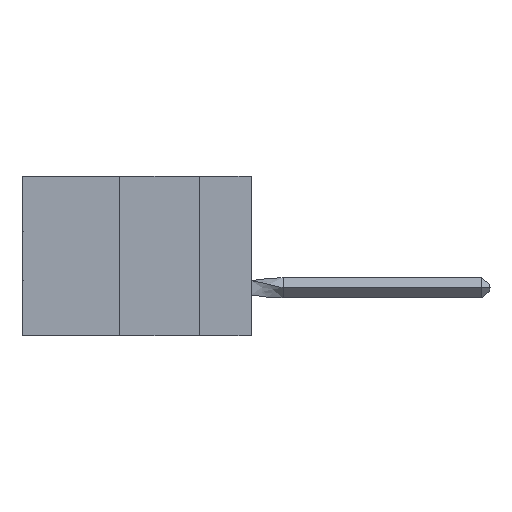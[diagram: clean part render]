
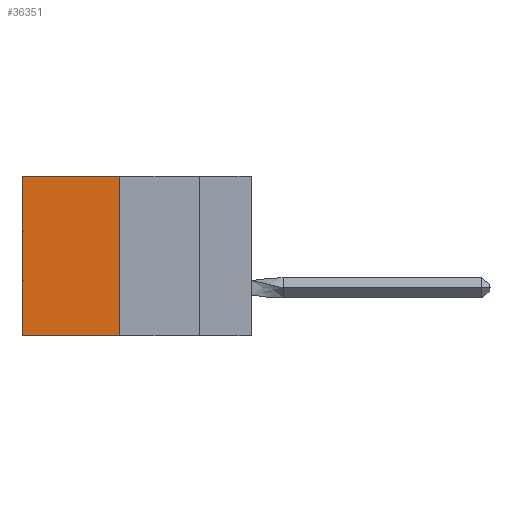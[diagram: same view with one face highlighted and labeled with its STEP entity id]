
A CAD part, left-side view. The second image highlights one B-rep face of the part: STEP entity #36351.
In plain terms, the highlighted planar face has unit normal (-1, 0, 0).
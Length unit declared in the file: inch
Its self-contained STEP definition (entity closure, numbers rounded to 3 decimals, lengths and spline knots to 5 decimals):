
#51 = CARTESIAN_POINT ( 'NONE',  ( 0.305, 0.72, -0.5 ) ) ;
#473 = EDGE_CURVE ( 'NONE', #9166, #6131, #24667, .T. ) ;
#812 = FACE_OUTER_BOUND ( 'NONE', #2274, .T. ) ;
#2274 = EDGE_LOOP ( 'NONE', ( #14143, #43478, #26600, #22146 ) ) ;
#3530 = CARTESIAN_POINT ( 'NONE',  ( 0.305, 0.413, 0. ) ) ;
#4498 = LINE ( 'NONE', #8764, #38368 ) ;
#6131 = VERTEX_POINT ( 'NONE', #32258 ) ;
#6392 = AXIS2_PLACEMENT_3D ( 'NONE', #42616, #46285, #28176 ) ;
#6401 = VERTEX_POINT ( 'NONE', #26428 ) ;
#6738 = DIRECTION ( 'NONE',  ( 0., 1., 0. ) ) ;
#6821 = LINE ( 'NONE', #3530, #35655 ) ;
#8726 = EDGE_CURVE ( 'NONE', #13160, #6131, #26101, .T. ) ;
#8764 = CARTESIAN_POINT ( 'NONE',  ( 0.305, 0.413, -0.5 ) ) ;
#9166 = VERTEX_POINT ( 'NONE', #20437 ) ;
#9474 = EDGE_CURVE ( 'NONE', #6401, #13160, #6821, .T. ) ;
#13160 = VERTEX_POINT ( 'NONE', #33735 ) ;
#13871 = VECTOR ( 'NONE', #6738, 39.37008 ) ;
#14143 = ORIENTED_EDGE ( 'NONE', *, *, #8726, .T. ) ;
#16470 = VECTOR ( 'NONE', #25133, 39.37008 ) ;
#17262 = CARTESIAN_POINT ( 'NONE',  ( 0.305, 0.413, -0.5 ) ) ;
#20437 = CARTESIAN_POINT ( 'NONE',  ( 0.305, 0.413, -0.5 ) ) ;
#22146 = ORIENTED_EDGE ( 'NONE', *, *, #9474, .T. ) ;
#24667 = LINE ( 'NONE', #17262, #13871 ) ;
#25133 = DIRECTION ( 'NONE',  ( 0., 0., -1. ) ) ;
#26101 = LINE ( 'NONE', #51, #16470 ) ;
#26428 = CARTESIAN_POINT ( 'NONE',  ( 0.305, 0.413, 0. ) ) ;
#26600 = ORIENTED_EDGE ( 'NONE', *, *, #39027, .F. ) ;
#28176 = DIRECTION ( 'NONE',  ( 0., 0., -1. ) ) ;
#32258 = CARTESIAN_POINT ( 'NONE',  ( 0.305, 0.72, -0.5 ) ) ;
#33735 = CARTESIAN_POINT ( 'NONE',  ( 0.305, 0.72, 0. ) ) ;
#35655 = VECTOR ( 'NONE', #43355, 39.37008 ) ;
#36351 = ADVANCED_FACE ( 'NONE', ( #812 ), #38954, .F. ) ;
#38368 = VECTOR ( 'NONE', #45007, 39.37008 ) ;
#38954 = PLANE ( 'NONE',  #6392 ) ;
#39027 = EDGE_CURVE ( 'NONE', #6401, #9166, #4498, .T. ) ;
#42616 = CARTESIAN_POINT ( 'NONE',  ( 0.305, 0.413, -0.5 ) ) ;
#43355 = DIRECTION ( 'NONE',  ( 0., 1., 0. ) ) ;
#43478 = ORIENTED_EDGE ( 'NONE', *, *, #473, .F. ) ;
#45007 = DIRECTION ( 'NONE',  ( 0., 0., -1. ) ) ;
#46285 = DIRECTION ( 'NONE',  ( 1., 0., 0. ) ) ;
